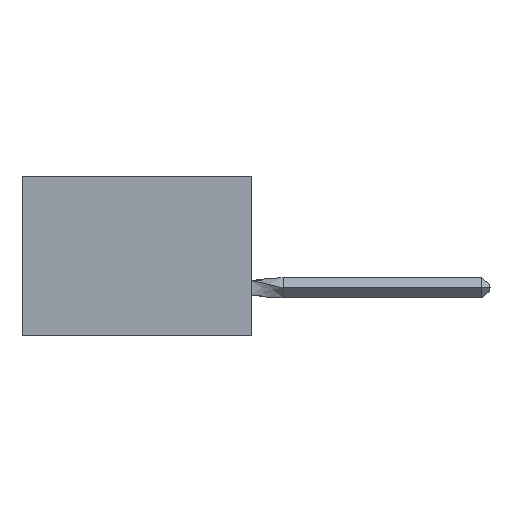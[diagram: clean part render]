
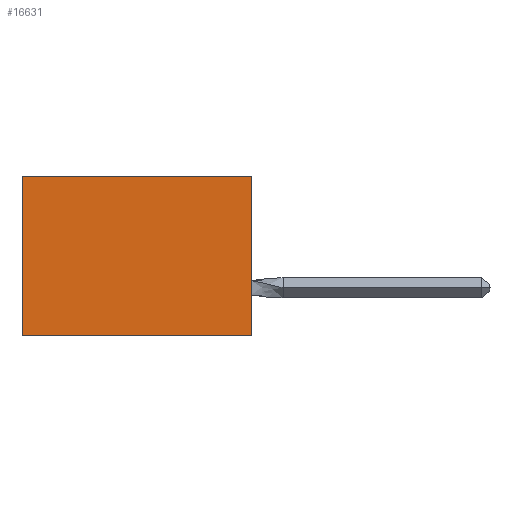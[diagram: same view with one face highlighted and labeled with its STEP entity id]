
A CAD part, left-side view. The second image highlights one B-rep face of the part: STEP entity #16631.
In plain terms, the highlighted planar face has unit normal (-1, 0, 0).
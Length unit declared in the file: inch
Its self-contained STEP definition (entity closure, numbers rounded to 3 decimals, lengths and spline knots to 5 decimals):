
#598 = EDGE_LOOP ( 'NONE', ( #18735, #23276, #13796, #14502 ) ) ;
#2508 = EDGE_CURVE ( 'NONE', #40372, #23519, #27293, .T. ) ;
#2704 = VERTEX_POINT ( 'NONE', #42230 ) ;
#3493 = VECTOR ( 'NONE', #38010, 39.37008 ) ;
#3723 = DIRECTION ( 'NONE',  ( 0., 1., 0. ) ) ;
#5054 = AXIS2_PLACEMENT_3D ( 'NONE', #26102, #33145, #36265 ) ;
#5821 = CARTESIAN_POINT ( 'NONE',  ( 0.305, 0., -0.5 ) ) ;
#9047 = CARTESIAN_POINT ( 'NONE',  ( 0.305, 0.72, 0. ) ) ;
#9412 = DIRECTION ( 'NONE',  ( 0., 0., -1. ) ) ;
#10093 = CARTESIAN_POINT ( 'NONE',  ( 0.305, 0., -0.5 ) ) ;
#13110 = EDGE_CURVE ( 'NONE', #40372, #20440, #18865, .T. ) ;
#13796 = ORIENTED_EDGE ( 'NONE', *, *, #13110, .F. ) ;
#14502 = ORIENTED_EDGE ( 'NONE', *, *, #2508, .T. ) ;
#16370 = LINE ( 'NONE', #19739, #37488 ) ;
#16631 = ADVANCED_FACE ( 'NONE', ( #27511 ), #35985, .F. ) ;
#17471 = LINE ( 'NONE', #10093, #36506 ) ;
#18735 = ORIENTED_EDGE ( 'NONE', *, *, #26849, .T. ) ;
#18865 = LINE ( 'NONE', #31228, #3493 ) ;
#18985 = CARTESIAN_POINT ( 'NONE',  ( 0.305, 0., 0. ) ) ;
#19739 = CARTESIAN_POINT ( 'NONE',  ( 0.305, 0.72, -0.5 ) ) ;
#20440 = VERTEX_POINT ( 'NONE', #5821 ) ;
#21859 = CARTESIAN_POINT ( 'NONE',  ( 0.305, 0., 0. ) ) ;
#22383 = DIRECTION ( 'NONE',  ( 0., 1., 0. ) ) ;
#23276 = ORIENTED_EDGE ( 'NONE', *, *, #29602, .F. ) ;
#23519 = VERTEX_POINT ( 'NONE', #9047 ) ;
#26102 = CARTESIAN_POINT ( 'NONE',  ( 0.305, 0., -0.5 ) ) ;
#26849 = EDGE_CURVE ( 'NONE', #23519, #2704, #16370, .T. ) ;
#27293 = LINE ( 'NONE', #18985, #34183 ) ;
#27511 = FACE_OUTER_BOUND ( 'NONE', #598, .T. ) ;
#29602 = EDGE_CURVE ( 'NONE', #20440, #2704, #17471, .T. ) ;
#31228 = CARTESIAN_POINT ( 'NONE',  ( 0.305, 0., -0.5 ) ) ;
#33145 = DIRECTION ( 'NONE',  ( 1., 0., 0. ) ) ;
#34183 = VECTOR ( 'NONE', #22383, 39.37008 ) ;
#35985 = PLANE ( 'NONE',  #5054 ) ;
#36265 = DIRECTION ( 'NONE',  ( 0., 0., -1. ) ) ;
#36506 = VECTOR ( 'NONE', #3723, 39.37008 ) ;
#37488 = VECTOR ( 'NONE', #9412, 39.37008 ) ;
#38010 = DIRECTION ( 'NONE',  ( 0., 0., -1. ) ) ;
#40372 = VERTEX_POINT ( 'NONE', #21859 ) ;
#42230 = CARTESIAN_POINT ( 'NONE',  ( 0.305, 0.72, -0.5 ) ) ;
